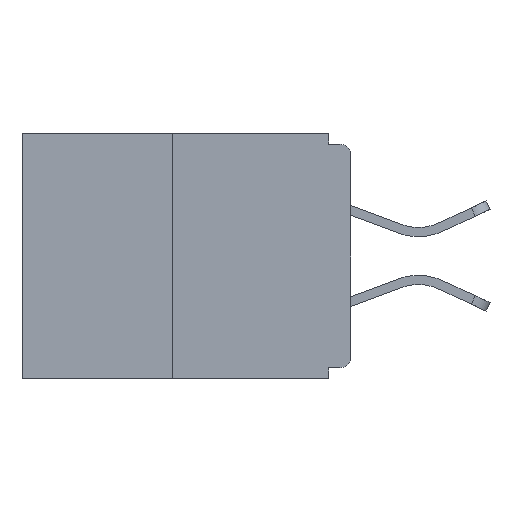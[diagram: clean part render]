
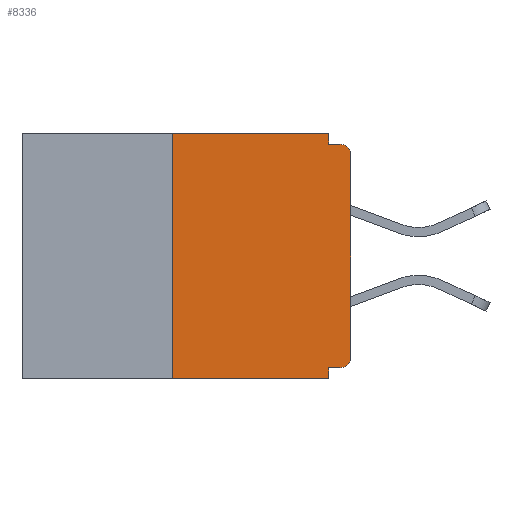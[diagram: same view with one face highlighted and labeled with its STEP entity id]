
A CAD part, left-side view. The second image highlights one B-rep face of the part: STEP entity #8336.
In plain terms, the highlighted planar face has unit normal (-1, 0, 0).
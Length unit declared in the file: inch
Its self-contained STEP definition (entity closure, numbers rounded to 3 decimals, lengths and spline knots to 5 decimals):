
#462 = LINE ( 'NONE', #8547, #10937 ) ;
#530 = DIRECTION ( 'NONE',  ( 0., 0., -1. ) ) ;
#677 = DIRECTION ( 'NONE',  ( 0., 0., -1. ) ) ;
#1088 = ORIENTED_EDGE ( 'NONE', *, *, #11612, .F. ) ;
#1141 = ORIENTED_EDGE ( 'NONE', *, *, #5094, .T. ) ;
#1203 = EDGE_CURVE ( 'NONE', #1247, #2781, #14740, .T. ) ;
#1247 = VERTEX_POINT ( 'NONE', #2732 ) ;
#1574 = CARTESIAN_POINT ( 'NONE',  ( 0., 0.46, -0.343 ) ) ;
#1929 = VECTOR ( 'NONE', #3395, 39.37008 ) ;
#2074 = VECTOR ( 'NONE', #11788, 39.37008 ) ;
#2131 = AXIS2_PLACEMENT_3D ( 'NONE', #6570, #5550, #13643 ) ;
#2570 = LINE ( 'NONE', #3590, #8786 ) ;
#2641 = EDGE_CURVE ( 'NONE', #8411, #6211, #462, .T. ) ;
#2732 = CARTESIAN_POINT ( 'NONE',  ( 0., 0.015, -0.328 ) ) ;
#2781 = VERTEX_POINT ( 'NONE', #15082 ) ;
#2815 = ORIENTED_EDGE ( 'NONE', *, *, #4624, .T. ) ;
#2886 = CIRCLE ( 'NONE', #2131, 0.015 ) ;
#2922 = DIRECTION ( 'NONE',  ( 1., 0., 0. ) ) ;
#2998 = DIRECTION ( 'NONE',  ( 0., 0., -1. ) ) ;
#3395 = DIRECTION ( 'NONE',  ( 0., -1., 0. ) ) ;
#3590 = CARTESIAN_POINT ( 'NONE',  ( 0., 0.25, 0. ) ) ;
#3726 = ORIENTED_EDGE ( 'NONE', *, *, #2641, .F. ) ;
#3908 = DIRECTION ( 'NONE',  ( 0., -1., 0. ) ) ;
#3911 = EDGE_LOOP ( 'NONE', ( #5814, #1088, #8737, #5400, #5483, #1141, #8731, #2815, #3726, #6647 ) ) ;
#4092 = EDGE_CURVE ( 'NONE', #14785, #11051, #10485, .T. ) ;
#4303 = VERTEX_POINT ( 'NONE', #7858 ) ;
#4469 = CARTESIAN_POINT ( 'NONE',  ( 0., 0.25, 0. ) ) ;
#4576 = CARTESIAN_POINT ( 'NONE',  ( 0., 0.46, 0. ) ) ;
#4624 = EDGE_CURVE ( 'NONE', #4303, #6211, #5303, .T. ) ;
#4658 = VECTOR ( 'NONE', #12497, 39.37008 ) ;
#5030 = CARTESIAN_POINT ( 'NONE',  ( 0., 0.031, 0. ) ) ;
#5094 = EDGE_CURVE ( 'NONE', #1247, #13292, #2886, .T. ) ;
#5276 = CARTESIAN_POINT ( 'NONE',  ( 0., 0.031, -0.015 ) ) ;
#5303 = CIRCLE ( 'NONE', #7278, 0.015 ) ;
#5400 = ORIENTED_EDGE ( 'NONE', *, *, #14897, .F. ) ;
#5483 = ORIENTED_EDGE ( 'NONE', *, *, #1203, .F. ) ;
#5550 = DIRECTION ( 'NONE',  ( -1., 0., 0. ) ) ;
#5566 = CARTESIAN_POINT ( 'NONE',  ( 0., 0.015, -0.03 ) ) ;
#5713 = EDGE_CURVE ( 'NONE', #11051, #8411, #14842, .T. ) ;
#5814 = ORIENTED_EDGE ( 'NONE', *, *, #4092, .F. ) ;
#5874 = LINE ( 'NONE', #10849, #2074 ) ;
#6211 = VERTEX_POINT ( 'NONE', #14824 ) ;
#6336 = EDGE_CURVE ( 'NONE', #13292, #4303, #14904, .T. ) ;
#6570 = CARTESIAN_POINT ( 'NONE',  ( 0., 0.015, -0.313 ) ) ;
#6593 = DIRECTION ( 'NONE',  ( -1., 0., 0. ) ) ;
#6645 = VECTOR ( 'NONE', #2998, 39.37008 ) ;
#6647 = ORIENTED_EDGE ( 'NONE', *, *, #5713, .F. ) ;
#7278 = AXIS2_PLACEMENT_3D ( 'NONE', #5566, #6593, #677 ) ;
#7603 = CARTESIAN_POINT ( 'NONE',  ( 0., 0.031, -0.343 ) ) ;
#7635 = VECTOR ( 'NONE', #13635, 39.37008 ) ;
#7729 = VERTEX_POINT ( 'NONE', #7603 ) ;
#7807 = CARTESIAN_POINT ( 'NONE',  ( 0., 0., 0. ) ) ;
#7858 = CARTESIAN_POINT ( 'NONE',  ( 0., 0., -0.03 ) ) ;
#7974 = CARTESIAN_POINT ( 'NONE',  ( 0., 0.031, 0. ) ) ;
#8336 = ADVANCED_FACE ( 'NONE', ( #8340 ), #13817, .F. ) ;
#8340 = FACE_OUTER_BOUND ( 'NONE', #3911, .T. ) ;
#8411 = VERTEX_POINT ( 'NONE', #5276 ) ;
#8547 = CARTESIAN_POINT ( 'NONE',  ( 0., 0., -0.015 ) ) ;
#8572 = LINE ( 'NONE', #1574, #10902 ) ;
#8731 = ORIENTED_EDGE ( 'NONE', *, *, #6336, .T. ) ;
#8737 = ORIENTED_EDGE ( 'NONE', *, *, #13041, .T. ) ;
#8786 = VECTOR ( 'NONE', #9661, 39.37008 ) ;
#9661 = DIRECTION ( 'NONE',  ( 0., 0., 1. ) ) ;
#9817 = CARTESIAN_POINT ( 'NONE',  ( 0., 0., -0.328 ) ) ;
#10485 = LINE ( 'NONE', #4576, #1929 ) ;
#10849 = CARTESIAN_POINT ( 'NONE',  ( 0., 0.031, -0.343 ) ) ;
#10902 = VECTOR ( 'NONE', #3908, 39.37008 ) ;
#10922 = AXIS2_PLACEMENT_3D ( 'NONE', #11193, #2922, #530 ) ;
#10937 = VECTOR ( 'NONE', #13311, 39.37008 ) ;
#11051 = VERTEX_POINT ( 'NONE', #7974 ) ;
#11193 = CARTESIAN_POINT ( 'NONE',  ( 0., 0.46, 0. ) ) ;
#11401 = VERTEX_POINT ( 'NONE', #13422 ) ;
#11612 = EDGE_CURVE ( 'NONE', #11401, #14785, #2570, .T. ) ;
#11788 = DIRECTION ( 'NONE',  ( 0., 0., -1. ) ) ;
#12497 = DIRECTION ( 'NONE',  ( 0., 0., 1. ) ) ;
#13041 = EDGE_CURVE ( 'NONE', #11401, #7729, #8572, .T. ) ;
#13292 = VERTEX_POINT ( 'NONE', #15335 ) ;
#13311 = DIRECTION ( 'NONE',  ( 0., -1., 0. ) ) ;
#13422 = CARTESIAN_POINT ( 'NONE',  ( 0., 0.25, -0.343 ) ) ;
#13635 = DIRECTION ( 'NONE',  ( 0., 1., 0. ) ) ;
#13643 = DIRECTION ( 'NONE',  ( 0., 0., -1. ) ) ;
#13817 = PLANE ( 'NONE',  #10922 ) ;
#14740 = LINE ( 'NONE', #9817, #7635 ) ;
#14785 = VERTEX_POINT ( 'NONE', #4469 ) ;
#14824 = CARTESIAN_POINT ( 'NONE',  ( 0., 0.015, -0.015 ) ) ;
#14842 = LINE ( 'NONE', #5030, #6645 ) ;
#14897 = EDGE_CURVE ( 'NONE', #2781, #7729, #5874, .T. ) ;
#14904 = LINE ( 'NONE', #7807, #4658 ) ;
#15082 = CARTESIAN_POINT ( 'NONE',  ( 0., 0.031, -0.328 ) ) ;
#15335 = CARTESIAN_POINT ( 'NONE',  ( 0., 0., -0.313 ) ) ;
